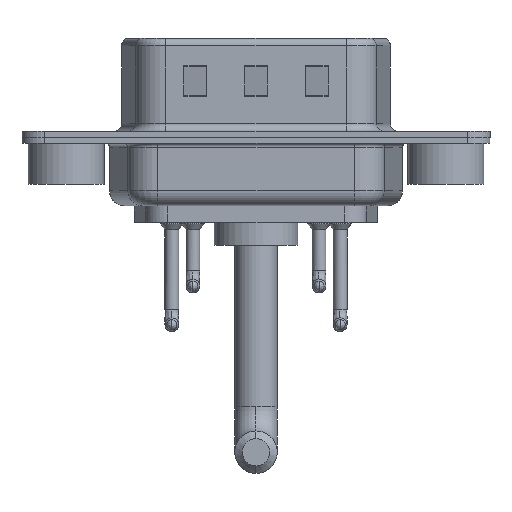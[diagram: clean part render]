
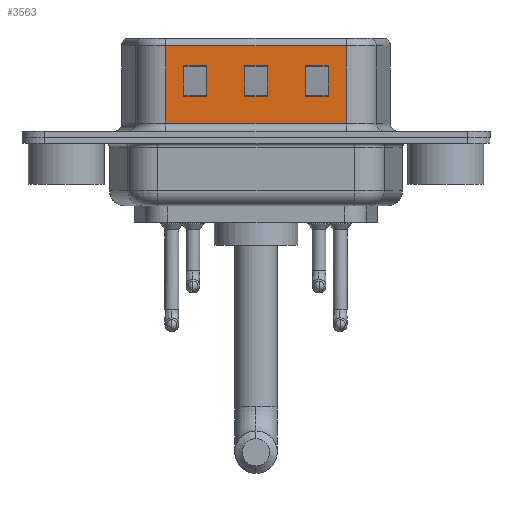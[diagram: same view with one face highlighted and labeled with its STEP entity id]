
A CAD part, front view. The second image highlights one B-rep face of the part: STEP entity #3563.
In plain terms, the highlighted planar face has unit normal (0, -1, 0).
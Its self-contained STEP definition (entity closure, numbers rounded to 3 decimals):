
#79 = ORIENTED_EDGE ( 'NONE', *, *, #11238, .T. ) ;
#145 = FACE_OUTER_BOUND ( 'NONE', #19296, .T. ) ;
#578 = CARTESIAN_POINT ( 'NONE',  ( 13.25, -4.55, 4.705 ) ) ;
#646 = CARTESIAN_POINT ( 'NONE',  ( 18.451, -4.55, 0.9 ) ) ;
#752 = CARTESIAN_POINT ( 'NONE',  ( 6.549, -4.55, 6.02 ) ) ;
#828 = CARTESIAN_POINT ( 'NONE',  ( 15.75, -4.55, 4.705 ) ) ;
#1020 = VECTOR ( 'NONE', #4485, 1000. ) ;
#1645 = CARTESIAN_POINT ( 'NONE',  ( 17.25, -4.55, 6.52 ) ) ;
#1794 = CARTESIAN_POINT ( 'NONE',  ( 22.451, -4.55, 4.705 ) ) ;
#2016 = CARTESIAN_POINT ( 'NONE',  ( 7.75, -4.55, 2.705 ) ) ;
#2089 = CARTESIAN_POINT ( 'NONE',  ( 11.75, -4.55, 6.52 ) ) ;
#2681 = ORIENTED_EDGE ( 'NONE', *, *, #14107, .T. ) ;
#2772 = DIRECTION ( 'NONE',  ( 0., 0., 1. ) ) ;
#2798 = FACE_BOUND ( 'NONE', #15430, .T. ) ;
#3036 = CARTESIAN_POINT ( 'NONE',  ( 17.25, -4.55, 4.705 ) ) ;
#3204 = CARTESIAN_POINT ( 'NONE',  ( 9.25, -4.55, 4.705 ) ) ;
#3247 = VECTOR ( 'NONE', #13508, 1000. ) ;
#3255 = CARTESIAN_POINT ( 'NONE',  ( 6.549, -4.55, 0.9 ) ) ;
#3414 = VECTOR ( 'NONE', #6195, 1000. ) ;
#3562 = EDGE_CURVE ( 'NONE', #11917, #19231, #16433, .T. ) ;
#3563 = ADVANCED_FACE ( 'NONE', ( #10238, #2798, #13592, #145 ), #18473, .F. ) ;
#3691 = VERTEX_POINT ( 'NONE', #18565 ) ;
#3977 = ORIENTED_EDGE ( 'NONE', *, *, #19010, .T. ) ;
#4135 = EDGE_CURVE ( 'NONE', #10384, #16142, #16697, .T. ) ;
#4278 = CARTESIAN_POINT ( 'NONE',  ( 18.451, -4.55, 6.52 ) ) ;
#4290 = LINE ( 'NONE', #10256, #10587 ) ;
#4478 = DIRECTION ( 'NONE',  ( 0., 0., -1. ) ) ;
#4485 = DIRECTION ( 'NONE',  ( 0., 0., -1. ) ) ;
#4502 = EDGE_CURVE ( 'NONE', #5836, #8392, #18469, .T. ) ;
#4510 = LINE ( 'NONE', #16668, #6495 ) ;
#4687 = CARTESIAN_POINT ( 'NONE',  ( 9.25, -4.55, 2.705 ) ) ;
#4868 = EDGE_CURVE ( 'NONE', #19316, #17957, #15712, .T. ) ;
#4989 = VECTOR ( 'NONE', #10909, 1000. ) ;
#5407 = EDGE_CURVE ( 'NONE', #16995, #8491, #4510, .T. ) ;
#5441 = CARTESIAN_POINT ( 'NONE',  ( 11.75, -4.55, 2.705 ) ) ;
#5522 = VERTEX_POINT ( 'NONE', #578 ) ;
#5777 = VECTOR ( 'NONE', #6358, 1000. ) ;
#5836 = VERTEX_POINT ( 'NONE', #10348 ) ;
#5846 = EDGE_CURVE ( 'NONE', #17957, #5522, #4290, .T. ) ;
#6195 = DIRECTION ( 'NONE',  ( 1., 0., 0. ) ) ;
#6222 = DIRECTION ( 'NONE',  ( 0., 1., 0. ) ) ;
#6240 = CARTESIAN_POINT ( 'NONE',  ( 11.75, -4.55, 4.705 ) ) ;
#6358 = DIRECTION ( 'NONE',  ( 0., 0., -1. ) ) ;
#6477 = DIRECTION ( 'NONE',  ( -1., 0., 0. ) ) ;
#6495 = VECTOR ( 'NONE', #9208, 1000. ) ;
#6540 = EDGE_LOOP ( 'NONE', ( #79, #14578, #19175, #17471 ) ) ;
#6986 = ORIENTED_EDGE ( 'NONE', *, *, #5407, .T. ) ;
#7002 = CARTESIAN_POINT ( 'NONE',  ( 18.451, -4.55, 6.02 ) ) ;
#7024 = CARTESIAN_POINT ( 'NONE',  ( 13.25, -4.55, 6.52 ) ) ;
#7097 = VERTEX_POINT ( 'NONE', #2016 ) ;
#7244 = LINE ( 'NONE', #7636, #9419 ) ;
#7345 = DIRECTION ( 'NONE',  ( -1., 0., 0. ) ) ;
#7510 = CARTESIAN_POINT ( 'NONE',  ( 7.75, -4.55, 6.52 ) ) ;
#7593 = CARTESIAN_POINT ( 'NONE',  ( 18.451, -4.55, 6.02 ) ) ;
#7636 = CARTESIAN_POINT ( 'NONE',  ( 14.451, -4.55, 2.705 ) ) ;
#7991 = EDGE_CURVE ( 'NONE', #5522, #3691, #12634, .T. ) ;
#8165 = EDGE_CURVE ( 'NONE', #7097, #5836, #16051, .T. ) ;
#8392 = VERTEX_POINT ( 'NONE', #3204 ) ;
#8491 = VERTEX_POINT ( 'NONE', #646 ) ;
#8639 = ORIENTED_EDGE ( 'NONE', *, *, #13724, .T. ) ;
#8644 = LINE ( 'NONE', #9825, #13446 ) ;
#8650 = ORIENTED_EDGE ( 'NONE', *, *, #14702, .F. ) ;
#8678 = AXIS2_PLACEMENT_3D ( 'NONE', #9547, #6222, #14071 ) ;
#8785 = CARTESIAN_POINT ( 'NONE',  ( 6.549, -4.55, 6.52 ) ) ;
#9208 = DIRECTION ( 'NONE',  ( 1., 0., 0. ) ) ;
#9419 = VECTOR ( 'NONE', #7345, 1000. ) ;
#9547 = CARTESIAN_POINT ( 'NONE',  ( 18.451, -4.55, 6.52 ) ) ;
#9614 = LINE ( 'NONE', #12390, #17189 ) ;
#9825 = CARTESIAN_POINT ( 'NONE',  ( 15.75, -4.55, 6.52 ) ) ;
#10234 = ORIENTED_EDGE ( 'NONE', *, *, #5846, .T. ) ;
#10238 = FACE_BOUND ( 'NONE', #6540, .T. ) ;
#10256 = CARTESIAN_POINT ( 'NONE',  ( 18.451, -4.55, 4.705 ) ) ;
#10348 = CARTESIAN_POINT ( 'NONE',  ( 7.75, -4.55, 4.705 ) ) ;
#10351 = LINE ( 'NONE', #1645, #1020 ) ;
#10384 = VERTEX_POINT ( 'NONE', #828 ) ;
#10587 = VECTOR ( 'NONE', #16546, 1000. ) ;
#10810 = LINE ( 'NONE', #12107, #14442 ) ;
#10909 = DIRECTION ( 'NONE',  ( 0., 0., 1. ) ) ;
#11068 = ORIENTED_EDGE ( 'NONE', *, *, #7991, .T. ) ;
#11238 = EDGE_CURVE ( 'NONE', #8392, #19074, #18326, .T. ) ;
#11432 = ORIENTED_EDGE ( 'NONE', *, *, #17763, .T. ) ;
#11917 = VERTEX_POINT ( 'NONE', #7002 ) ;
#11924 = LINE ( 'NONE', #4278, #18154 ) ;
#12107 = CARTESIAN_POINT ( 'NONE',  ( 22.451, -4.55, 2.705 ) ) ;
#12261 = VERTEX_POINT ( 'NONE', #15602 ) ;
#12390 = CARTESIAN_POINT ( 'NONE',  ( 18.451, -4.55, 2.705 ) ) ;
#12634 = LINE ( 'NONE', #7024, #13873 ) ;
#12876 = ORIENTED_EDGE ( 'NONE', *, *, #4868, .T. ) ;
#13025 = DIRECTION ( 'NONE',  ( 0., 0., -1. ) ) ;
#13115 = VECTOR ( 'NONE', #16524, 1000. ) ;
#13446 = VECTOR ( 'NONE', #2772, 1000. ) ;
#13493 = DIRECTION ( 'NONE',  ( -1., 0., 0. ) ) ;
#13508 = DIRECTION ( 'NONE',  ( 0., 0., 1. ) ) ;
#13592 = FACE_BOUND ( 'NONE', #18331, .T. ) ;
#13682 = DIRECTION ( 'NONE',  ( -1., 0., 0. ) ) ;
#13724 = EDGE_CURVE ( 'NONE', #14077, #10384, #8644, .T. ) ;
#13788 = CARTESIAN_POINT ( 'NONE',  ( 14.451, -4.55, 4.705 ) ) ;
#13833 = CARTESIAN_POINT ( 'NONE',  ( 9.25, -4.55, 6.52 ) ) ;
#13873 = VECTOR ( 'NONE', #13025, 1000. ) ;
#14071 = DIRECTION ( 'NONE',  ( -1., 0., 0. ) ) ;
#14077 = VERTEX_POINT ( 'NONE', #16974 ) ;
#14107 = EDGE_CURVE ( 'NONE', #3691, #19316, #9614, .T. ) ;
#14442 = VECTOR ( 'NONE', #13682, 1000. ) ;
#14578 = ORIENTED_EDGE ( 'NONE', *, *, #16124, .T. ) ;
#14604 = ORIENTED_EDGE ( 'NONE', *, *, #3562, .T. ) ;
#14702 = EDGE_CURVE ( 'NONE', #11917, #8491, #11924, .T. ) ;
#15430 = EDGE_LOOP ( 'NONE', ( #3977, #16469, #8639, #17832 ) ) ;
#15602 = CARTESIAN_POINT ( 'NONE',  ( 17.25, -4.55, 2.705 ) ) ;
#15712 = LINE ( 'NONE', #2089, #4989 ) ;
#16051 = LINE ( 'NONE', #7510, #3247 ) ;
#16124 = EDGE_CURVE ( 'NONE', #19074, #7097, #7244, .T. ) ;
#16142 = VERTEX_POINT ( 'NONE', #3036 ) ;
#16433 = LINE ( 'NONE', #7593, #17148 ) ;
#16469 = ORIENTED_EDGE ( 'NONE', *, *, #16523, .T. ) ;
#16523 = EDGE_CURVE ( 'NONE', #12261, #14077, #10810, .T. ) ;
#16524 = DIRECTION ( 'NONE',  ( 1., 0., 0. ) ) ;
#16546 = DIRECTION ( 'NONE',  ( 1., 0., 0. ) ) ;
#16668 = CARTESIAN_POINT ( 'NONE',  ( 18.451, -4.55, 0.9 ) ) ;
#16693 = VECTOR ( 'NONE', #4478, 1000. ) ;
#16697 = LINE ( 'NONE', #1794, #3414 ) ;
#16974 = CARTESIAN_POINT ( 'NONE',  ( 15.75, -4.55, 2.705 ) ) ;
#16995 = VERTEX_POINT ( 'NONE', #3255 ) ;
#17148 = VECTOR ( 'NONE', #13493, 1000. ) ;
#17189 = VECTOR ( 'NONE', #6477, 1000. ) ;
#17471 = ORIENTED_EDGE ( 'NONE', *, *, #4502, .T. ) ;
#17763 = EDGE_CURVE ( 'NONE', #19231, #16995, #19371, .T. ) ;
#17832 = ORIENTED_EDGE ( 'NONE', *, *, #4135, .T. ) ;
#17957 = VERTEX_POINT ( 'NONE', #6240 ) ;
#18154 = VECTOR ( 'NONE', #19267, 1000. ) ;
#18326 = LINE ( 'NONE', #13833, #5777 ) ;
#18331 = EDGE_LOOP ( 'NONE', ( #10234, #11068, #2681, #12876 ) ) ;
#18469 = LINE ( 'NONE', #13788, #13115 ) ;
#18473 = PLANE ( 'NONE',  #8678 ) ;
#18565 = CARTESIAN_POINT ( 'NONE',  ( 13.25, -4.55, 2.705 ) ) ;
#19010 = EDGE_CURVE ( 'NONE', #16142, #12261, #10351, .T. ) ;
#19074 = VERTEX_POINT ( 'NONE', #4687 ) ;
#19175 = ORIENTED_EDGE ( 'NONE', *, *, #8165, .T. ) ;
#19231 = VERTEX_POINT ( 'NONE', #752 ) ;
#19267 = DIRECTION ( 'NONE',  ( 0., 0., -1. ) ) ;
#19296 = EDGE_LOOP ( 'NONE', ( #8650, #14604, #11432, #6986 ) ) ;
#19316 = VERTEX_POINT ( 'NONE', #5441 ) ;
#19371 = LINE ( 'NONE', #8785, #16693 ) ;
